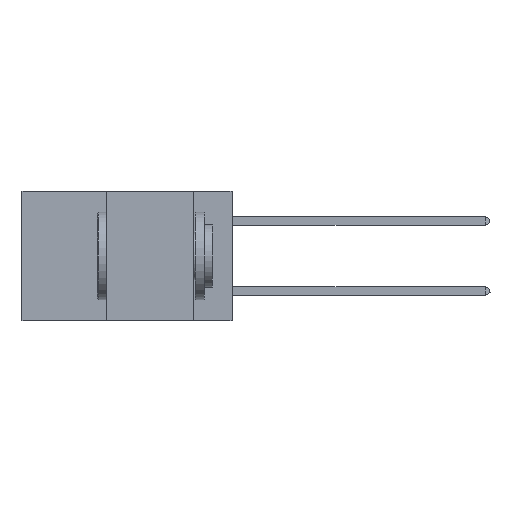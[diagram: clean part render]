
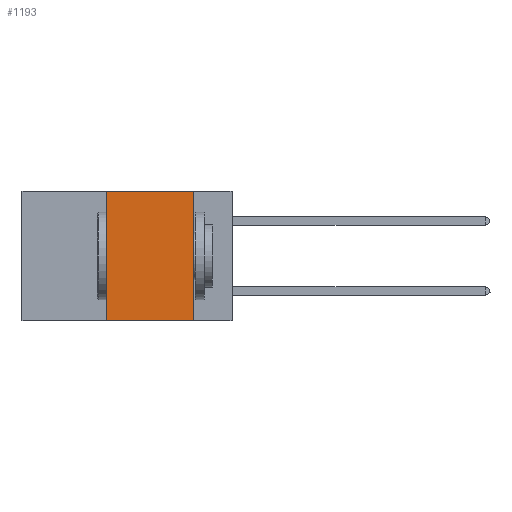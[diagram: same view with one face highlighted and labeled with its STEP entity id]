
A CAD part, left-side view. The second image highlights one B-rep face of the part: STEP entity #1193.
In plain terms, the highlighted planar face has unit normal (-1, 0, 0).
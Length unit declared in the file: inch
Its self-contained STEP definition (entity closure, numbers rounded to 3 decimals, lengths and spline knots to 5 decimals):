
#32 = VERTEX_POINT ( 'NONE', #10632 ) ;
#573 = CARTESIAN_POINT ( 'NONE',  ( 0., 0.11, 0. ) ) ;
#782 = EDGE_CURVE ( 'NONE', #7756, #3600, #11959, .T. ) ;
#1193 = ADVANCED_FACE ( 'NONE', ( #6538 ), #2306, .F. ) ;
#2190 = ORIENTED_EDGE ( 'NONE', *, *, #3711, .F. ) ;
#2218 = CARTESIAN_POINT ( 'NONE',  ( 0., 0.11, -0.37 ) ) ;
#2306 = PLANE ( 'NONE',  #6528 ) ;
#2650 = LINE ( 'NONE', #8089, #3682 ) ;
#3600 = VERTEX_POINT ( 'NONE', #2218 ) ;
#3682 = VECTOR ( 'NONE', #8971, 39.37008 ) ;
#3711 = EDGE_CURVE ( 'NONE', #32, #7756, #7205, .T. ) ;
#4261 = DIRECTION ( 'NONE',  ( 0., 0., -1. ) ) ;
#4344 = DIRECTION ( 'NONE',  ( 0., -1., 0. ) ) ;
#4391 = DIRECTION ( 'NONE',  ( 1., 0., 0. ) ) ;
#4571 = ORIENTED_EDGE ( 'NONE', *, *, #782, .F. ) ;
#4858 = LINE ( 'NONE', #10132, #9719 ) ;
#5515 = DIRECTION ( 'NONE',  ( 0., -1., 0. ) ) ;
#5574 = EDGE_CURVE ( 'NONE', #6259, #32, #2650, .T. ) ;
#6240 = EDGE_LOOP ( 'NONE', ( #4571, #2190, #9290, #11201 ) ) ;
#6259 = VERTEX_POINT ( 'NONE', #11024 ) ;
#6260 = DIRECTION ( 'NONE',  ( 0., 0., -1. ) ) ;
#6306 = EDGE_CURVE ( 'NONE', #6259, #3600, #4858, .T. ) ;
#6528 = AXIS2_PLACEMENT_3D ( 'NONE', #9857, #4391, #4261 ) ;
#6538 = FACE_OUTER_BOUND ( 'NONE', #6240, .T. ) ;
#6633 = CARTESIAN_POINT ( 'NONE',  ( 0., 0.11, 0. ) ) ;
#7205 = LINE ( 'NONE', #11705, #9142 ) ;
#7756 = VERTEX_POINT ( 'NONE', #6633 ) ;
#7849 = VECTOR ( 'NONE', #6260, 39.37008 ) ;
#8089 = CARTESIAN_POINT ( 'NONE',  ( 0., 0.36, 0. ) ) ;
#8971 = DIRECTION ( 'NONE',  ( 0., 0., 1. ) ) ;
#9142 = VECTOR ( 'NONE', #4344, 39.37008 ) ;
#9290 = ORIENTED_EDGE ( 'NONE', *, *, #5574, .F. ) ;
#9719 = VECTOR ( 'NONE', #5515, 39.37008 ) ;
#9857 = CARTESIAN_POINT ( 'NONE',  ( 0., 0.6, 0. ) ) ;
#10132 = CARTESIAN_POINT ( 'NONE',  ( 0., 0.6, -0.37 ) ) ;
#10632 = CARTESIAN_POINT ( 'NONE',  ( 0., 0.36, 0. ) ) ;
#11024 = CARTESIAN_POINT ( 'NONE',  ( 0., 0.36, -0.37 ) ) ;
#11201 = ORIENTED_EDGE ( 'NONE', *, *, #6306, .T. ) ;
#11705 = CARTESIAN_POINT ( 'NONE',  ( 0., 0.6, 0. ) ) ;
#11959 = LINE ( 'NONE', #573, #7849 ) ;
